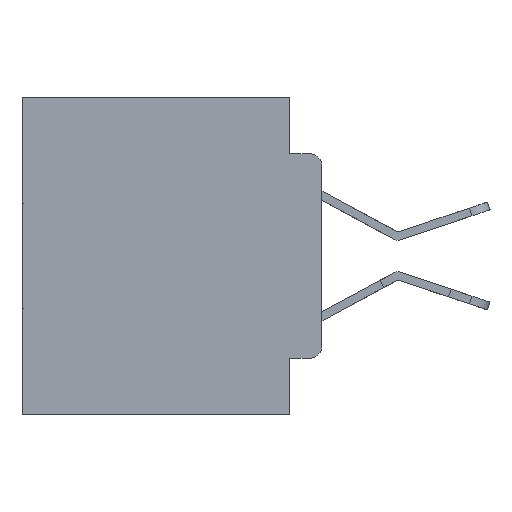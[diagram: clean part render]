
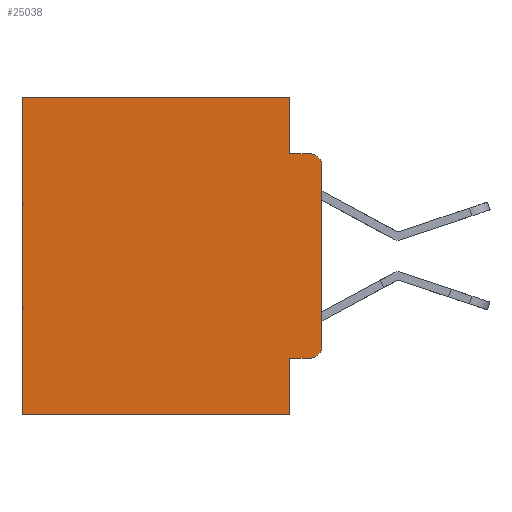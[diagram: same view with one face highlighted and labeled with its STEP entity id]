
A CAD part, left-side view. The second image highlights one B-rep face of the part: STEP entity #25038.
In plain terms, the highlighted planar face has unit normal (-1, 0, 0).
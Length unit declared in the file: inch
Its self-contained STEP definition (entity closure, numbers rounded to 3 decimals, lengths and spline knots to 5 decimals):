
#623 = VERTEX_POINT ( 'NONE', #29213 ) ;
#672 = VERTEX_POINT ( 'NONE', #8399 ) ;
#1407 = EDGE_CURVE ( 'NONE', #13114, #25045, #10288, .T. ) ;
#1521 = LINE ( 'NONE', #25253, #6434 ) ;
#1728 = CARTESIAN_POINT ( 'NONE',  ( 0.298, 0.051, -0.4115 ) ) ;
#1841 = EDGE_CURVE ( 'NONE', #672, #14087, #29416, .T. ) ;
#2385 = AXIS2_PLACEMENT_3D ( 'NONE', #4369, #20733, #6803 ) ;
#2843 = VERTEX_POINT ( 'NONE', #28348 ) ;
#3203 = VECTOR ( 'NONE', #25573, 39.37008 ) ;
#3891 = DIRECTION ( 'NONE',  ( 0., -1., 0. ) ) ;
#4273 = CARTESIAN_POINT ( 'NONE',  ( 0.298, 0.02, -0.0885 ) ) ;
#4369 = CARTESIAN_POINT ( 'NONE',  ( 0.298, 0.02, -0.3915 ) ) ;
#4513 = DIRECTION ( 'NONE',  ( 0., 1., 0. ) ) ;
#4769 = CIRCLE ( 'NONE', #29649, 0.02 ) ;
#4841 = CARTESIAN_POINT ( 'NONE',  ( 0.298, 0.051, 0. ) ) ;
#4938 = CARTESIAN_POINT ( 'NONE',  ( 0.298, 0.051, -0.0885 ) ) ;
#5031 = VECTOR ( 'NONE', #14342, 39.37008 ) ;
#5956 = EDGE_CURVE ( 'NONE', #15995, #623, #18751, .T. ) ;
#6434 = VECTOR ( 'NONE', #27553, 39.37008 ) ;
#6803 = DIRECTION ( 'NONE',  ( 0., 0., -1. ) ) ;
#7118 = VERTEX_POINT ( 'NONE', #10466 ) ;
#7279 = VECTOR ( 'NONE', #4513, 39.37008 ) ;
#7858 = CARTESIAN_POINT ( 'NONE',  ( 0.298, 0.051, -0.5 ) ) ;
#7945 = EDGE_CURVE ( 'NONE', #7118, #24427, #16861, .T. ) ;
#7986 = FACE_OUTER_BOUND ( 'NONE', #26717, .T. ) ;
#8173 = DIRECTION ( 'NONE',  ( 0., 0., -1. ) ) ;
#8399 = CARTESIAN_POINT ( 'NONE',  ( 0.298, 0.051, -0.4115 ) ) ;
#9187 = CARTESIAN_POINT ( 'NONE',  ( 0.298, 0., 0. ) ) ;
#9436 = LINE ( 'NONE', #24386, #27874 ) ;
#10066 = AXIS2_PLACEMENT_3D ( 'NONE', #9187, #25382, #11497 ) ;
#10088 = CARTESIAN_POINT ( 'NONE',  ( 0.298, 0., -0.3915 ) ) ;
#10118 = ORIENTED_EDGE ( 'NONE', *, *, #20723, .T. ) ;
#10288 = LINE ( 'NONE', #18127, #3203 ) ;
#10466 = CARTESIAN_POINT ( 'NONE',  ( 0.298, 0., -0.1085 ) ) ;
#10587 = VERTEX_POINT ( 'NONE', #7858 ) ;
#10983 = VECTOR ( 'NONE', #3891, 39.37008 ) ;
#11155 = CARTESIAN_POINT ( 'NONE',  ( 0.298, 0.02, -0.1085 ) ) ;
#11295 = LINE ( 'NONE', #21239, #5031 ) ;
#11422 = DIRECTION ( 'NONE',  ( 0., 0., -1. ) ) ;
#11430 = VECTOR ( 'NONE', #11422, 39.37008 ) ;
#11497 = DIRECTION ( 'NONE',  ( 0., 0., -1. ) ) ;
#11692 = CARTESIAN_POINT ( 'NONE',  ( 0.298, 0., 0. ) ) ;
#11971 = EDGE_CURVE ( 'NONE', #623, #2843, #9436, .T. ) ;
#13114 = VERTEX_POINT ( 'NONE', #4938 ) ;
#13469 = DIRECTION ( 'NONE',  ( 0., 0., -1. ) ) ;
#14087 = VERTEX_POINT ( 'NONE', #26940 ) ;
#14185 = LINE ( 'NONE', #25504, #7279 ) ;
#14342 = DIRECTION ( 'NONE',  ( 0., 0., -1. ) ) ;
#14958 = EDGE_CURVE ( 'NONE', #10587, #2843, #14185, .T. ) ;
#15055 = ORIENTED_EDGE ( 'NONE', *, *, #27464, .T. ) ;
#15995 = VERTEX_POINT ( 'NONE', #4841 ) ;
#16861 = LINE ( 'NONE', #25308, #11430 ) ;
#18127 = CARTESIAN_POINT ( 'NONE',  ( 0.298, 0.051, -0.0885 ) ) ;
#18751 = LINE ( 'NONE', #11692, #23499 ) ;
#20723 = EDGE_CURVE ( 'NONE', #14087, #24427, #23136, .T. ) ;
#20733 = DIRECTION ( 'NONE',  ( -1., 0., 0. ) ) ;
#20734 = PLANE ( 'NONE',  #10066 ) ;
#21239 = CARTESIAN_POINT ( 'NONE',  ( 0.298, 0.051, 0. ) ) ;
#22908 = ORIENTED_EDGE ( 'NONE', *, *, #30125, .F. ) ;
#23136 = CIRCLE ( 'NONE', #2385, 0.02 ) ;
#23499 = VECTOR ( 'NONE', #30141, 39.37008 ) ;
#24386 = CARTESIAN_POINT ( 'NONE',  ( 0.298, 0.473, 0. ) ) ;
#24427 = VERTEX_POINT ( 'NONE', #10088 ) ;
#24628 = ORIENTED_EDGE ( 'NONE', *, *, #5956, .T. ) ;
#25038 = ADVANCED_FACE ( 'NONE', ( #7986 ), #20734, .F. ) ;
#25045 = VERTEX_POINT ( 'NONE', #4273 ) ;
#25122 = ORIENTED_EDGE ( 'NONE', *, *, #14958, .F. ) ;
#25253 = CARTESIAN_POINT ( 'NONE',  ( 0.298, 0.051, 0. ) ) ;
#25308 = CARTESIAN_POINT ( 'NONE',  ( 0.298, 0., 0. ) ) ;
#25339 = ORIENTED_EDGE ( 'NONE', *, *, #7945, .F. ) ;
#25382 = DIRECTION ( 'NONE',  ( 1., 0., 0. ) ) ;
#25504 = CARTESIAN_POINT ( 'NONE',  ( 0.298, 0., -0.5 ) ) ;
#25553 = EDGE_CURVE ( 'NONE', #15995, #13114, #1521, .T. ) ;
#25573 = DIRECTION ( 'NONE',  ( 0., -1., 0. ) ) ;
#25672 = ORIENTED_EDGE ( 'NONE', *, *, #11971, .T. ) ;
#25859 = ORIENTED_EDGE ( 'NONE', *, *, #25553, .F. ) ;
#25929 = ORIENTED_EDGE ( 'NONE', *, *, #1407, .F. ) ;
#26717 = EDGE_LOOP ( 'NONE', ( #25339, #15055, #25929, #25859, #24628, #25672, #25122, #22908, #29838, #10118 ) ) ;
#26940 = CARTESIAN_POINT ( 'NONE',  ( 0.298, 0.02, -0.4115 ) ) ;
#27313 = DIRECTION ( 'NONE',  ( -1., 0., 0. ) ) ;
#27464 = EDGE_CURVE ( 'NONE', #7118, #25045, #4769, .T. ) ;
#27553 = DIRECTION ( 'NONE',  ( 0., 0., -1. ) ) ;
#27874 = VECTOR ( 'NONE', #8173, 39.37008 ) ;
#28348 = CARTESIAN_POINT ( 'NONE',  ( 0.298, 0.473, -0.5 ) ) ;
#29213 = CARTESIAN_POINT ( 'NONE',  ( 0.298, 0.473, 0. ) ) ;
#29416 = LINE ( 'NONE', #1728, #10983 ) ;
#29649 = AXIS2_PLACEMENT_3D ( 'NONE', #11155, #27313, #13469 ) ;
#29838 = ORIENTED_EDGE ( 'NONE', *, *, #1841, .T. ) ;
#30125 = EDGE_CURVE ( 'NONE', #672, #10587, #11295, .T. ) ;
#30141 = DIRECTION ( 'NONE',  ( 0., 1., 0. ) ) ;
